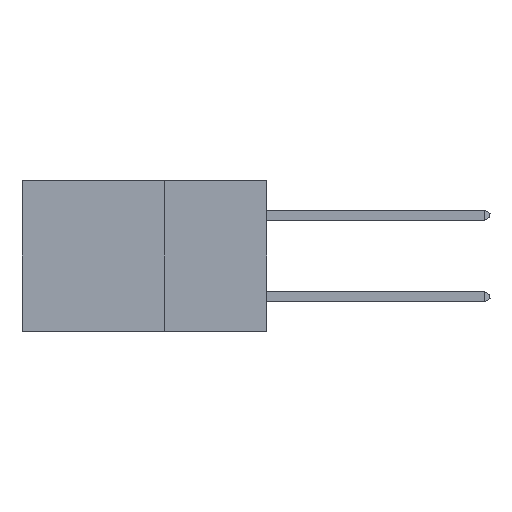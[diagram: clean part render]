
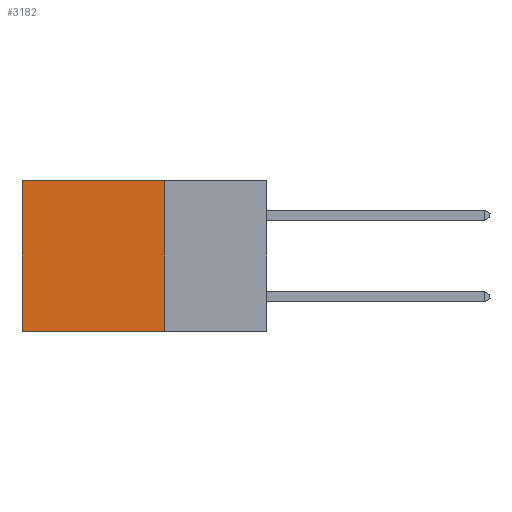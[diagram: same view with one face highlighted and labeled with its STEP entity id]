
A CAD part, left-side view. The second image highlights one B-rep face of the part: STEP entity #3182.
In plain terms, the highlighted planar face has unit normal (-1, 0, 0).
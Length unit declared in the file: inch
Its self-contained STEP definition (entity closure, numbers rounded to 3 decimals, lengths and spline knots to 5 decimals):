
#492 = VECTOR ( 'NONE', #805, 39.37008 ) ;
#805 = DIRECTION ( 'NONE',  ( 0., 1., 0. ) ) ;
#1299 = AXIS2_PLACEMENT_3D ( 'NONE', #9386, #9319, #9316 ) ;
#1743 = CARTESIAN_POINT ( 'NONE',  ( 0.2875, 0.6, 0. ) ) ;
#1793 = CARTESIAN_POINT ( 'NONE',  ( 0.2875, 0.25, 0. ) ) ;
#1874 = EDGE_CURVE ( 'NONE', #14447, #13759, #6926, .T. ) ;
#1895 = DIRECTION ( 'NONE',  ( 0., 0., -1. ) ) ;
#2060 = VECTOR ( 'NONE', #9828, 39.37008 ) ;
#2391 = VERTEX_POINT ( 'NONE', #4226 ) ;
#3182 = ADVANCED_FACE ( 'NONE', ( #11030 ), #9416, .F. ) ;
#4226 = CARTESIAN_POINT ( 'NONE',  ( 0.2875, 0.25, 0. ) ) ;
#5332 = EDGE_LOOP ( 'NONE', ( #6511, #13624, #8226, #5775 ) ) ;
#5536 = DIRECTION ( 'NONE',  ( 0., 0., -1. ) ) ;
#5775 = ORIENTED_EDGE ( 'NONE', *, *, #11047, .T. ) ;
#6425 = CARTESIAN_POINT ( 'NONE',  ( 0.2875, 0.25, -0.37 ) ) ;
#6455 = LINE ( 'NONE', #1793, #15212 ) ;
#6511 = ORIENTED_EDGE ( 'NONE', *, *, #1874, .T. ) ;
#6926 = LINE ( 'NONE', #1743, #10012 ) ;
#7538 = CARTESIAN_POINT ( 'NONE',  ( 0.2875, 0.6, -0.37 ) ) ;
#8226 = ORIENTED_EDGE ( 'NONE', *, *, #12629, .F. ) ;
#8231 = CARTESIAN_POINT ( 'NONE',  ( 0.2875, 0.25, -0.37 ) ) ;
#8680 = CARTESIAN_POINT ( 'NONE',  ( 0.2875, 0.25, 0. ) ) ;
#9316 = DIRECTION ( 'NONE',  ( 0., 0., -1. ) ) ;
#9319 = DIRECTION ( 'NONE',  ( 1., 0., 0. ) ) ;
#9386 = CARTESIAN_POINT ( 'NONE',  ( 0.2875, 0.25, 0. ) ) ;
#9416 = PLANE ( 'NONE',  #1299 ) ;
#9828 = DIRECTION ( 'NONE',  ( 0., 1., 0. ) ) ;
#10012 = VECTOR ( 'NONE', #1895, 39.37008 ) ;
#10267 = LINE ( 'NONE', #8231, #492 ) ;
#11030 = FACE_OUTER_BOUND ( 'NONE', #5332, .T. ) ;
#11047 = EDGE_CURVE ( 'NONE', #2391, #14447, #11927, .T. ) ;
#11927 = LINE ( 'NONE', #8680, #2060 ) ;
#12345 = CARTESIAN_POINT ( 'NONE',  ( 0.2875, 0.6, 0. ) ) ;
#12455 = VERTEX_POINT ( 'NONE', #6425 ) ;
#12629 = EDGE_CURVE ( 'NONE', #2391, #12455, #6455, .T. ) ;
#13624 = ORIENTED_EDGE ( 'NONE', *, *, #14019, .F. ) ;
#13759 = VERTEX_POINT ( 'NONE', #7538 ) ;
#14019 = EDGE_CURVE ( 'NONE', #12455, #13759, #10267, .T. ) ;
#14447 = VERTEX_POINT ( 'NONE', #12345 ) ;
#15212 = VECTOR ( 'NONE', #5536, 39.37008 ) ;
